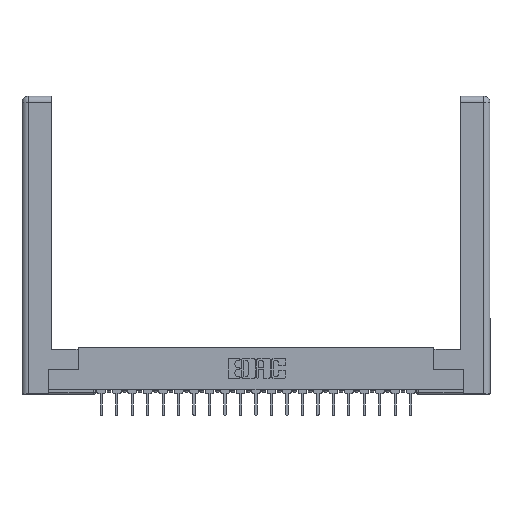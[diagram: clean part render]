
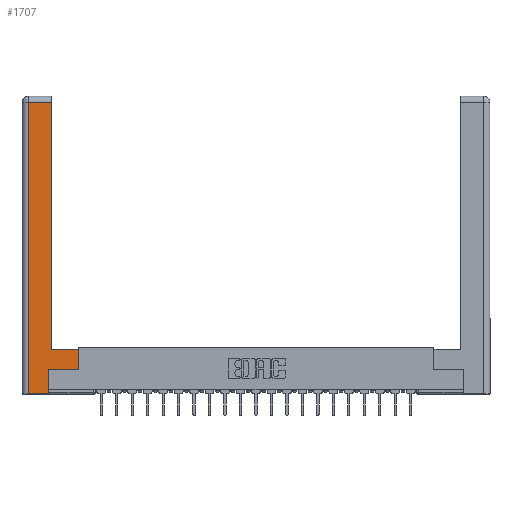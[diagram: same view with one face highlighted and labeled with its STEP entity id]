
A CAD part, top view. The second image highlights one B-rep face of the part: STEP entity #1707.
In plain terms, the highlighted planar face has unit normal (0, 0, 1).
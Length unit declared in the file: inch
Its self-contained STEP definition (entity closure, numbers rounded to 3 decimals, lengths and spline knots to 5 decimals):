
#56 = CARTESIAN_POINT ( 'NONE',  ( 0.0615, 0., 0. ) ) ;
#217 = EDGE_CURVE ( 'NONE', #5387, #17787, #6009, .T. ) ;
#498 = CARTESIAN_POINT ( 'NONE',  ( 0.265, 0., 0. ) ) ;
#521 = EDGE_CURVE ( 'NONE', #12223, #18869, #5501, .T. ) ;
#581 = VERTEX_POINT ( 'NONE', #56 ) ;
#887 = ORIENTED_EDGE ( 'NONE', *, *, #521, .T. ) ;
#942 = VERTEX_POINT ( 'NONE', #23846 ) ;
#1250 = CARTESIAN_POINT ( 'NONE',  ( 0.565, 0.245, 0. ) ) ;
#1351 = ORIENTED_EDGE ( 'NONE', *, *, #5157, .T. ) ;
#1509 = DIRECTION ( 'NONE',  ( -1., 0., 0. ) ) ;
#1707 = ADVANCED_FACE ( 'NONE', ( #5146 ), #19911, .F. ) ;
#2925 = VECTOR ( 'NONE', #22762, 39.37008 ) ;
#2997 = CARTESIAN_POINT ( 'NONE',  ( 0.265, 0.245, 0. ) ) ;
#3021 = CARTESIAN_POINT ( 'NONE',  ( 0.565, 0.45, 0. ) ) ;
#3065 = CARTESIAN_POINT ( 'NONE',  ( 0.0615, 2.94, 0. ) ) ;
#3076 = CARTESIAN_POINT ( 'NONE',  ( 0.0615, 0., 0. ) ) ;
#3194 = LINE ( 'NONE', #3076, #11401 ) ;
#3321 = CARTESIAN_POINT ( 'NONE',  ( 0., 0., 0. ) ) ;
#4069 = AXIS2_PLACEMENT_3D ( 'NONE', #3321, #10703, #1509 ) ;
#4190 = CARTESIAN_POINT ( 'NONE',  ( 0.565, 0.245, 0. ) ) ;
#4305 = EDGE_CURVE ( 'NONE', #18869, #13331, #10976, .T. ) ;
#5146 = FACE_OUTER_BOUND ( 'NONE', #17753, .T. ) ;
#5157 = EDGE_CURVE ( 'NONE', #13331, #942, #9319, .T. ) ;
#5336 = DIRECTION ( 'NONE',  ( 1., 0., 0. ) ) ;
#5387 = VERTEX_POINT ( 'NONE', #10147 ) ;
#5501 = LINE ( 'NONE', #17966, #10692 ) ;
#6009 = LINE ( 'NONE', #4190, #12985 ) ;
#6437 = CARTESIAN_POINT ( 'NONE',  ( 0.295, 2.94, 0. ) ) ;
#6848 = ORIENTED_EDGE ( 'NONE', *, *, #217, .T. ) ;
#7177 = VECTOR ( 'NONE', #14757, 39.37008 ) ;
#7567 = DIRECTION ( 'NONE',  ( 1., 0., 0. ) ) ;
#7921 = ORIENTED_EDGE ( 'NONE', *, *, #4305, .T. ) ;
#8280 = VECTOR ( 'NONE', #9993, 39.37008 ) ;
#8999 = DIRECTION ( 'NONE',  ( -1., 0., 0. ) ) ;
#9214 = ORIENTED_EDGE ( 'NONE', *, *, #22713, .T. ) ;
#9319 = LINE ( 'NONE', #3065, #7177 ) ;
#9993 = DIRECTION ( 'NONE',  ( 0., 1., 0. ) ) ;
#10147 = CARTESIAN_POINT ( 'NONE',  ( 0.265, 0.245, 0. ) ) ;
#10692 = VECTOR ( 'NONE', #8999, 39.37008 ) ;
#10703 = DIRECTION ( 'NONE',  ( 0., 0., -1. ) ) ;
#10976 = LINE ( 'NONE', #18367, #8280 ) ;
#11401 = VECTOR ( 'NONE', #17846, 39.37008 ) ;
#12098 = VERTEX_POINT ( 'NONE', #498 ) ;
#12223 = VERTEX_POINT ( 'NONE', #3021 ) ;
#12985 = VECTOR ( 'NONE', #7567, 39.37008 ) ;
#13331 = VERTEX_POINT ( 'NONE', #6437 ) ;
#13524 = ORIENTED_EDGE ( 'NONE', *, *, #22265, .T. ) ;
#13964 = EDGE_CURVE ( 'NONE', #12098, #5387, #22956, .T. ) ;
#14757 = DIRECTION ( 'NONE',  ( -1., 0., 0. ) ) ;
#14763 = CARTESIAN_POINT ( 'NONE',  ( 0.265, 0., 0. ) ) ;
#14893 = ORIENTED_EDGE ( 'NONE', *, *, #13964, .T. ) ;
#14919 = EDGE_CURVE ( 'NONE', #17787, #12223, #15385, .T. ) ;
#15385 = LINE ( 'NONE', #19033, #2925 ) ;
#15716 = CARTESIAN_POINT ( 'NONE',  ( 0.295, 0.45, 0. ) ) ;
#15942 = DIRECTION ( 'NONE',  ( 0., 1., 0. ) ) ;
#17165 = ORIENTED_EDGE ( 'NONE', *, *, #14919, .T. ) ;
#17753 = EDGE_LOOP ( 'NONE', ( #7921, #1351, #13524, #9214, #14893, #6848, #17165, #887 ) ) ;
#17787 = VERTEX_POINT ( 'NONE', #1250 ) ;
#17846 = DIRECTION ( 'NONE',  ( 0., -1., 0. ) ) ;
#17966 = CARTESIAN_POINT ( 'NONE',  ( 0.295, 0.45, 0. ) ) ;
#18367 = CARTESIAN_POINT ( 'NONE',  ( 0.295, 3., 0. ) ) ;
#18399 = VECTOR ( 'NONE', #5336, 39.37008 ) ;
#18869 = VERTEX_POINT ( 'NONE', #15716 ) ;
#19033 = CARTESIAN_POINT ( 'NONE',  ( 0.565, 0.45, 0. ) ) ;
#19911 = PLANE ( 'NONE',  #4069 ) ;
#20566 = LINE ( 'NONE', #14763, #18399 ) ;
#21420 = VECTOR ( 'NONE', #15942, 39.37008 ) ;
#22265 = EDGE_CURVE ( 'NONE', #942, #581, #3194, .T. ) ;
#22713 = EDGE_CURVE ( 'NONE', #581, #12098, #20566, .T. ) ;
#22762 = DIRECTION ( 'NONE',  ( 0., 1., 0. ) ) ;
#22956 = LINE ( 'NONE', #2997, #21420 ) ;
#23846 = CARTESIAN_POINT ( 'NONE',  ( 0.0615, 2.94, 0. ) ) ;
